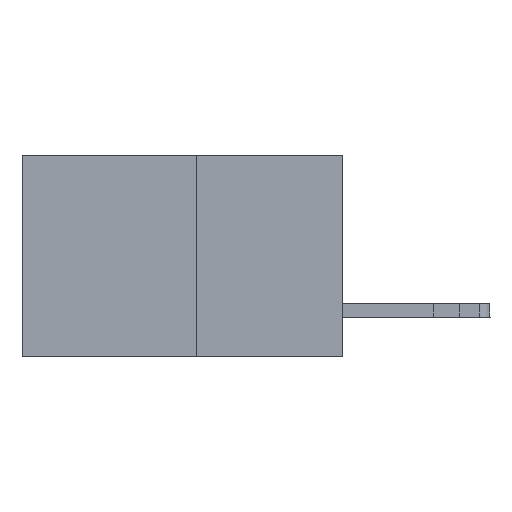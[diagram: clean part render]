
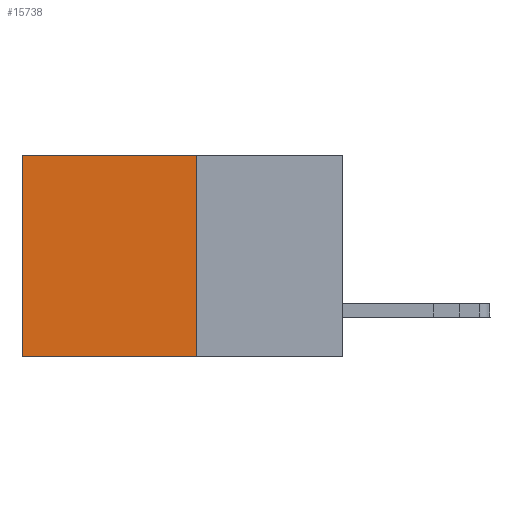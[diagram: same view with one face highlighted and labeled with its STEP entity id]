
A CAD part, left-side view. The second image highlights one B-rep face of the part: STEP entity #15738.
In plain terms, the highlighted planar face has unit normal (-1, 0, 0).
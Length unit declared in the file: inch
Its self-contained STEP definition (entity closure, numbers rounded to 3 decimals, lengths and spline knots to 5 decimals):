
#282 = CARTESIAN_POINT ( 'NONE',  ( 0.277, 0.27, 0. ) ) ;
#529 = DIRECTION ( 'NONE',  ( 1., 0., 0. ) ) ;
#749 = VECTOR ( 'NONE', #26536, 39.37008 ) ;
#1464 = CARTESIAN_POINT ( 'NONE',  ( 0.277, 0.27, -0.37 ) ) ;
#4318 = EDGE_CURVE ( 'NONE', #15991, #20441, #8493, .T. ) ;
#6084 = AXIS2_PLACEMENT_3D ( 'NONE', #12632, #529, #19347 ) ;
#7294 = ORIENTED_EDGE ( 'NONE', *, *, #20262, .F. ) ;
#8330 = CARTESIAN_POINT ( 'NONE',  ( 0.277, 0.27, -0.37 ) ) ;
#8493 = LINE ( 'NONE', #282, #16706 ) ;
#9114 = EDGE_CURVE ( 'NONE', #15392, #23669, #14007, .T. ) ;
#9703 = CARTESIAN_POINT ( 'NONE',  ( 0.277, 0.27, -0.37 ) ) ;
#10092 = VECTOR ( 'NONE', #15988, 39.37008 ) ;
#12497 = PLANE ( 'NONE',  #6084 ) ;
#12632 = CARTESIAN_POINT ( 'NONE',  ( 0.277, 0.27, -0.37 ) ) ;
#12723 = CARTESIAN_POINT ( 'NONE',  ( 0.277, 0.59, 0. ) ) ;
#13528 = CARTESIAN_POINT ( 'NONE',  ( 0.277, 0.59, -0.37 ) ) ;
#13930 = EDGE_LOOP ( 'NONE', ( #17527, #17882, #7294, #21795 ) ) ;
#14007 = LINE ( 'NONE', #9703, #10092 ) ;
#15392 = VERTEX_POINT ( 'NONE', #8330 ) ;
#15738 = ADVANCED_FACE ( 'NONE', ( #23134 ), #12497, .F. ) ;
#15988 = DIRECTION ( 'NONE',  ( 0., 1., 0. ) ) ;
#15991 = VERTEX_POINT ( 'NONE', #24494 ) ;
#16706 = VECTOR ( 'NONE', #25648, 39.37008 ) ;
#17527 = ORIENTED_EDGE ( 'NONE', *, *, #21941, .T. ) ;
#17882 = ORIENTED_EDGE ( 'NONE', *, *, #9114, .F. ) ;
#19347 = DIRECTION ( 'NONE',  ( 0., 0., -1. ) ) ;
#19859 = CARTESIAN_POINT ( 'NONE',  ( 0.277, 0.59, -0.37 ) ) ;
#20262 = EDGE_CURVE ( 'NONE', #15991, #15392, #20578, .T. ) ;
#20441 = VERTEX_POINT ( 'NONE', #12723 ) ;
#20578 = LINE ( 'NONE', #1464, #24278 ) ;
#21795 = ORIENTED_EDGE ( 'NONE', *, *, #4318, .T. ) ;
#21941 = EDGE_CURVE ( 'NONE', #20441, #23669, #26281, .T. ) ;
#23134 = FACE_OUTER_BOUND ( 'NONE', #13930, .T. ) ;
#23669 = VERTEX_POINT ( 'NONE', #13528 ) ;
#24278 = VECTOR ( 'NONE', #26961, 39.37008 ) ;
#24494 = CARTESIAN_POINT ( 'NONE',  ( 0.277, 0.27, 0. ) ) ;
#25648 = DIRECTION ( 'NONE',  ( 0., 1., 0. ) ) ;
#26281 = LINE ( 'NONE', #19859, #749 ) ;
#26536 = DIRECTION ( 'NONE',  ( 0., 0., -1. ) ) ;
#26961 = DIRECTION ( 'NONE',  ( 0., 0., -1. ) ) ;
